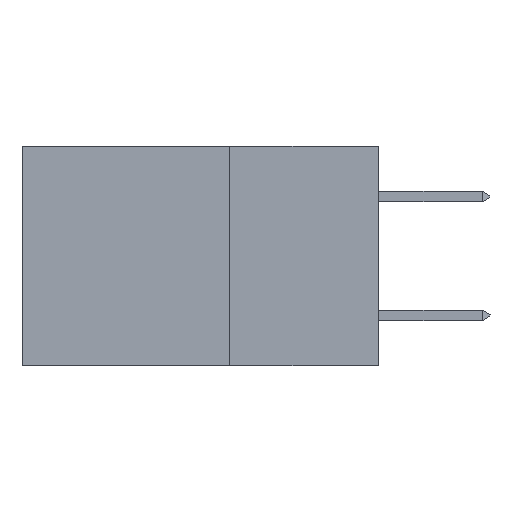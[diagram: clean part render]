
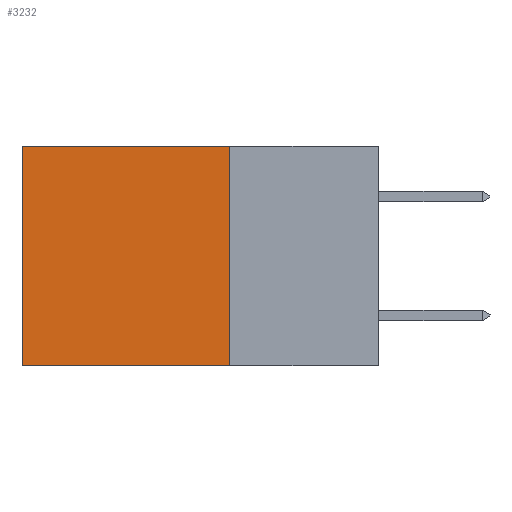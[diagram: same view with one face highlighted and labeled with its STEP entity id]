
A CAD part, left-side view. The second image highlights one B-rep face of the part: STEP entity #3232.
In plain terms, the highlighted planar face has unit normal (-1, 0, 0).
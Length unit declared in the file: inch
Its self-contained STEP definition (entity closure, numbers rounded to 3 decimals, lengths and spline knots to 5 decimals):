
#219 = CARTESIAN_POINT ( 'NONE',  ( 0.2615, 0.25, -0.37 ) ) ;
#283 = EDGE_CURVE ( 'NONE', #8806, #8988, #9117, .T. ) ;
#419 = VECTOR ( 'NONE', #11345, 39.37008 ) ;
#474 = EDGE_CURVE ( 'NONE', #4780, #6085, #4299, .T. ) ;
#566 = EDGE_LOOP ( 'NONE', ( #5541, #6786, #11118, #4933 ) ) ;
#770 = CARTESIAN_POINT ( 'NONE',  ( 0.2615, 0.25, 0. ) ) ;
#1125 = LINE ( 'NONE', #770, #419 ) ;
#1219 = CARTESIAN_POINT ( 'NONE',  ( 0.2615, 0.25, -0.37 ) ) ;
#2072 = DIRECTION ( 'NONE',  ( 1., 0., 0. ) ) ;
#2211 = CARTESIAN_POINT ( 'NONE',  ( 0.2615, 0.25, -0.37 ) ) ;
#2301 = AXIS2_PLACEMENT_3D ( 'NONE', #1219, #2072, #9201 ) ;
#2434 = CARTESIAN_POINT ( 'NONE',  ( 0.2615, 0.6, -0.37 ) ) ;
#3048 = VECTOR ( 'NONE', #9508, 39.37008 ) ;
#3107 = DIRECTION ( 'NONE',  ( 0., 0., -1. ) ) ;
#3232 = ADVANCED_FACE ( 'NONE', ( #9591 ), #6547, .F. ) ;
#4145 = VECTOR ( 'NONE', #3107, 39.37008 ) ;
#4299 = LINE ( 'NONE', #2211, #4145 ) ;
#4780 = VERTEX_POINT ( 'NONE', #10743 ) ;
#4933 = ORIENTED_EDGE ( 'NONE', *, *, #10748, .T. ) ;
#5541 = ORIENTED_EDGE ( 'NONE', *, *, #283, .T. ) ;
#5559 = VECTOR ( 'NONE', #10819, 39.37008 ) ;
#6085 = VERTEX_POINT ( 'NONE', #9396 ) ;
#6547 = PLANE ( 'NONE',  #2301 ) ;
#6786 = ORIENTED_EDGE ( 'NONE', *, *, #9904, .F. ) ;
#8642 = CARTESIAN_POINT ( 'NONE',  ( 0.2615, 0.6, -0.37 ) ) ;
#8806 = VERTEX_POINT ( 'NONE', #10269 ) ;
#8988 = VERTEX_POINT ( 'NONE', #8642 ) ;
#9117 = LINE ( 'NONE', #2434, #3048 ) ;
#9201 = DIRECTION ( 'NONE',  ( 0., 0., -1. ) ) ;
#9396 = CARTESIAN_POINT ( 'NONE',  ( 0.2615, 0.25, -0.37 ) ) ;
#9508 = DIRECTION ( 'NONE',  ( 0., 0., -1. ) ) ;
#9591 = FACE_OUTER_BOUND ( 'NONE', #566, .T. ) ;
#9904 = EDGE_CURVE ( 'NONE', #6085, #8988, #11046, .T. ) ;
#10269 = CARTESIAN_POINT ( 'NONE',  ( 0.2615, 0.6, 0. ) ) ;
#10743 = CARTESIAN_POINT ( 'NONE',  ( 0.2615, 0.25, 0. ) ) ;
#10748 = EDGE_CURVE ( 'NONE', #4780, #8806, #1125, .T. ) ;
#10819 = DIRECTION ( 'NONE',  ( 0., 1., 0. ) ) ;
#11046 = LINE ( 'NONE', #219, #5559 ) ;
#11118 = ORIENTED_EDGE ( 'NONE', *, *, #474, .F. ) ;
#11345 = DIRECTION ( 'NONE',  ( 0., 1., 0. ) ) ;
